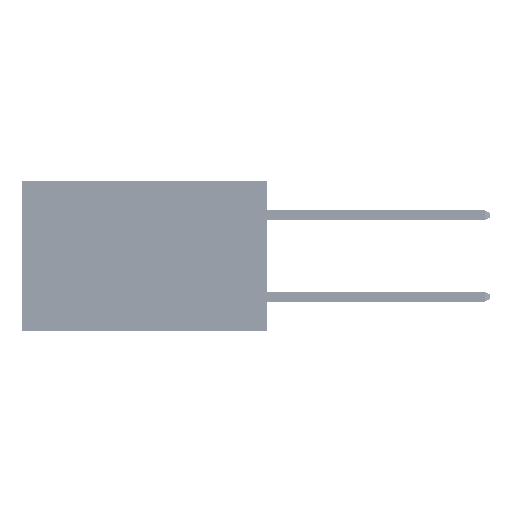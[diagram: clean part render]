
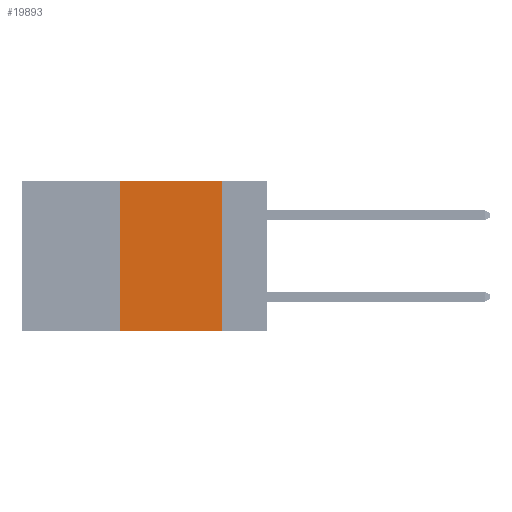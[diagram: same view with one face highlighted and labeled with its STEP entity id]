
A CAD part, left-side view. The second image highlights one B-rep face of the part: STEP entity #19893.
In plain terms, the highlighted planar face has unit normal (-1, 0, 0).
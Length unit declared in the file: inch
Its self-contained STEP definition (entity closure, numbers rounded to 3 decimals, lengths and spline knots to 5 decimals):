
#1713 = VERTEX_POINT ( 'NONE', #10394 ) ;
#2190 = VERTEX_POINT ( 'NONE', #12660 ) ;
#3523 = CARTESIAN_POINT ( 'NONE',  ( 0., 0.36, -0.37 ) ) ;
#3773 = LINE ( 'NONE', #39786, #29815 ) ;
#5033 = CARTESIAN_POINT ( 'NONE',  ( 0., 0.36, 0. ) ) ;
#6854 = CARTESIAN_POINT ( 'NONE',  ( 0., 0.6, -0.37 ) ) ;
#9047 = DIRECTION ( 'NONE',  ( 1., 0., 0. ) ) ;
#10169 = EDGE_CURVE ( 'NONE', #50788, #2190, #30528, .T. ) ;
#10331 = VECTOR ( 'NONE', #13016, 39.37008 ) ;
#10394 = CARTESIAN_POINT ( 'NONE',  ( 0., 0.11, -0.37 ) ) ;
#11338 = EDGE_CURVE ( 'NONE', #14041, #1713, #13059, .T. ) ;
#11554 = ORIENTED_EDGE ( 'NONE', *, *, #10169, .F. ) ;
#12660 = CARTESIAN_POINT ( 'NONE',  ( 0., 0.11, 0. ) ) ;
#12933 = PLANE ( 'NONE',  #47725 ) ;
#13016 = DIRECTION ( 'NONE',  ( 0., 0., 1. ) ) ;
#13059 = LINE ( 'NONE', #6854, #50520 ) ;
#14041 = VERTEX_POINT ( 'NONE', #3523 ) ;
#15400 = DIRECTION ( 'NONE',  ( 0., 0., -1. ) ) ;
#19893 = ADVANCED_FACE ( 'NONE', ( #32623 ), #12933, .F. ) ;
#21905 = EDGE_CURVE ( 'NONE', #2190, #1713, #3773, .T. ) ;
#26454 = EDGE_LOOP ( 'NONE', ( #50844, #11554, #47382, #48818 ) ) ;
#28721 = CARTESIAN_POINT ( 'NONE',  ( 0., 0.36, 0. ) ) ;
#29235 = VECTOR ( 'NONE', #47750, 39.37008 ) ;
#29815 = VECTOR ( 'NONE', #15400, 39.37008 ) ;
#30528 = LINE ( 'NONE', #44078, #29235 ) ;
#32623 = FACE_OUTER_BOUND ( 'NONE', #26454, .T. ) ;
#33896 = EDGE_CURVE ( 'NONE', #14041, #50788, #42086, .T. ) ;
#37669 = CARTESIAN_POINT ( 'NONE',  ( 0., 0.6, 0. ) ) ;
#39786 = CARTESIAN_POINT ( 'NONE',  ( 0., 0.11, 0. ) ) ;
#41395 = DIRECTION ( 'NONE',  ( 0., 0., -1. ) ) ;
#42086 = LINE ( 'NONE', #5033, #10331 ) ;
#44078 = CARTESIAN_POINT ( 'NONE',  ( 0., 0.6, 0. ) ) ;
#47382 = ORIENTED_EDGE ( 'NONE', *, *, #33896, .F. ) ;
#47725 = AXIS2_PLACEMENT_3D ( 'NONE', #37669, #9047, #41395 ) ;
#47750 = DIRECTION ( 'NONE',  ( 0., -1., 0. ) ) ;
#48818 = ORIENTED_EDGE ( 'NONE', *, *, #11338, .T. ) ;
#50520 = VECTOR ( 'NONE', #51184, 39.37008 ) ;
#50788 = VERTEX_POINT ( 'NONE', #28721 ) ;
#50844 = ORIENTED_EDGE ( 'NONE', *, *, #21905, .F. ) ;
#51184 = DIRECTION ( 'NONE',  ( 0., -1., 0. ) ) ;
